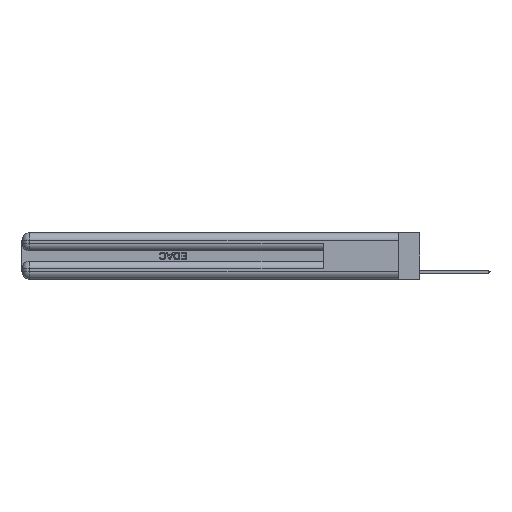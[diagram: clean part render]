
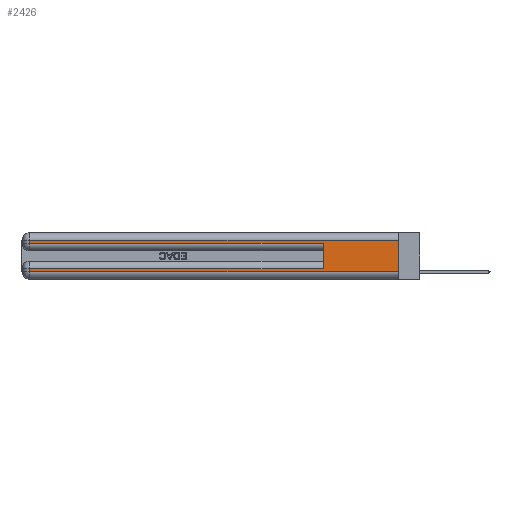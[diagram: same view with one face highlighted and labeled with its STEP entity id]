
A CAD part, left-side view. The second image highlights one B-rep face of the part: STEP entity #2426.
In plain terms, the highlighted planar face has unit normal (-1, 0, 0).
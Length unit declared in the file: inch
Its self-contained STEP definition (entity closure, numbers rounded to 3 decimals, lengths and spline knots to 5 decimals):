
#351 = CARTESIAN_POINT ( 'NONE',  ( 0., 0., 0.37 ) ) ;
#756 = VECTOR ( 'NONE', #15267, 39.37008 ) ;
#1898 = VECTOR ( 'NONE', #32781, 39.37008 ) ;
#2426 = ADVANCED_FACE ( 'NONE', ( #9090 ), #15568, .F. ) ;
#4268 = AXIS2_PLACEMENT_3D ( 'NONE', #351, #22808, #10258 ) ;
#5447 = ORIENTED_EDGE ( 'NONE', *, *, #29836, .F. ) ;
#5464 = VERTEX_POINT ( 'NONE', #7803 ) ;
#5858 = ORIENTED_EDGE ( 'NONE', *, *, #12553, .T. ) ;
#5859 = EDGE_CURVE ( 'NONE', #21022, #28348, #22028, .T. ) ;
#7019 = CARTESIAN_POINT ( 'NONE',  ( 0., 0., 0.37 ) ) ;
#7520 = ORIENTED_EDGE ( 'NONE', *, *, #13550, .T. ) ;
#7803 = CARTESIAN_POINT ( 'NONE',  ( 0., 2.94, 0.06 ) ) ;
#7831 = CARTESIAN_POINT ( 'NONE',  ( 0., 2.94, 0.285 ) ) ;
#8028 = LINE ( 'NONE', #7019, #25429 ) ;
#8912 = CARTESIAN_POINT ( 'NONE',  ( 0., 2.94, 0.31 ) ) ;
#8920 = ORIENTED_EDGE ( 'NONE', *, *, #22230, .F. ) ;
#9090 = FACE_OUTER_BOUND ( 'NONE', #22754, .T. ) ;
#9249 = LINE ( 'NONE', #18766, #12841 ) ;
#9746 = DIRECTION ( 'NONE',  ( 0., -1., 0. ) ) ;
#10250 = CARTESIAN_POINT ( 'NONE',  ( 0., 2.94, 0.37 ) ) ;
#10258 = DIRECTION ( 'NONE',  ( 0., 0., -1. ) ) ;
#10487 = ORIENTED_EDGE ( 'NONE', *, *, #15950, .T. ) ;
#10588 = DIRECTION ( 'NONE',  ( 0., 0., -1. ) ) ;
#12553 = EDGE_CURVE ( 'NONE', #5464, #17507, #20185, .T. ) ;
#12841 = VECTOR ( 'NONE', #23820, 39.37008 ) ;
#13314 = LINE ( 'NONE', #10250, #31914 ) ;
#13550 = EDGE_CURVE ( 'NONE', #28348, #5464, #22073, .T. ) ;
#13628 = ORIENTED_EDGE ( 'NONE', *, *, #5859, .T. ) ;
#15267 = DIRECTION ( 'NONE',  ( 0., -1., 0. ) ) ;
#15568 = PLANE ( 'NONE',  #4268 ) ;
#15698 = VERTEX_POINT ( 'NONE', #8912 ) ;
#15883 = ORIENTED_EDGE ( 'NONE', *, *, #25912, .T. ) ;
#15950 = EDGE_CURVE ( 'NONE', #15698, #29721, #13314, .T. ) ;
#16502 = CARTESIAN_POINT ( 'NONE',  ( 0., 0., 0.31 ) ) ;
#16601 = VECTOR ( 'NONE', #31085, 39.37008 ) ;
#17497 = CARTESIAN_POINT ( 'NONE',  ( 0., 0., 0.285 ) ) ;
#17507 = VERTEX_POINT ( 'NONE', #28150 ) ;
#18116 = EDGE_CURVE ( 'NONE', #29721, #24409, #30836, .T. ) ;
#18167 = VECTOR ( 'NONE', #9746, 39.37008 ) ;
#18248 = CARTESIAN_POINT ( 'NONE',  ( 0., 0., 0.06 ) ) ;
#18299 = ORIENTED_EDGE ( 'NONE', *, *, #18116, .T. ) ;
#18766 = CARTESIAN_POINT ( 'NONE',  ( 0., 0., 0.31 ) ) ;
#19584 = CARTESIAN_POINT ( 'NONE',  ( 0., 0., 0.085 ) ) ;
#20185 = LINE ( 'NONE', #18248, #756 ) ;
#20327 = CARTESIAN_POINT ( 'NONE',  ( 0., 2.94, 0.37 ) ) ;
#21022 = VERTEX_POINT ( 'NONE', #29365 ) ;
#21179 = CARTESIAN_POINT ( 'NONE',  ( 0., 0.6, 0.285 ) ) ;
#21243 = VECTOR ( 'NONE', #27261, 39.37008 ) ;
#22028 = LINE ( 'NONE', #19584, #21243 ) ;
#22073 = LINE ( 'NONE', #20327, #1898 ) ;
#22230 = EDGE_CURVE ( 'NONE', #24446, #17507, #8028, .T. ) ;
#22754 = EDGE_LOOP ( 'NONE', ( #8920, #15883, #10487, #18299, #5447, #13628, #7520, #5858 ) ) ;
#22808 = DIRECTION ( 'NONE',  ( 1., 0., 0. ) ) ;
#23820 = DIRECTION ( 'NONE',  ( 0., 1., 0. ) ) ;
#24409 = VERTEX_POINT ( 'NONE', #21179 ) ;
#24446 = VERTEX_POINT ( 'NONE', #16502 ) ;
#25429 = VECTOR ( 'NONE', #32518, 39.37008 ) ;
#25912 = EDGE_CURVE ( 'NONE', #24446, #15698, #9249, .T. ) ;
#27261 = DIRECTION ( 'NONE',  ( 0., 1., 0. ) ) ;
#28150 = CARTESIAN_POINT ( 'NONE',  ( 0., 0., 0.06 ) ) ;
#28348 = VERTEX_POINT ( 'NONE', #32415 ) ;
#28527 = CARTESIAN_POINT ( 'NONE',  ( 0., 0.6, 0.145 ) ) ;
#29365 = CARTESIAN_POINT ( 'NONE',  ( 0., 0.6, 0.085 ) ) ;
#29721 = VERTEX_POINT ( 'NONE', #7831 ) ;
#29836 = EDGE_CURVE ( 'NONE', #21022, #24409, #30066, .T. ) ;
#30066 = LINE ( 'NONE', #28527, #16601 ) ;
#30836 = LINE ( 'NONE', #17497, #18167 ) ;
#31085 = DIRECTION ( 'NONE',  ( 0., 0., 1. ) ) ;
#31914 = VECTOR ( 'NONE', #10588, 39.37008 ) ;
#32415 = CARTESIAN_POINT ( 'NONE',  ( 0., 2.94, 0.085 ) ) ;
#32518 = DIRECTION ( 'NONE',  ( 0., 0., -1. ) ) ;
#32781 = DIRECTION ( 'NONE',  ( 0., 0., -1. ) ) ;
